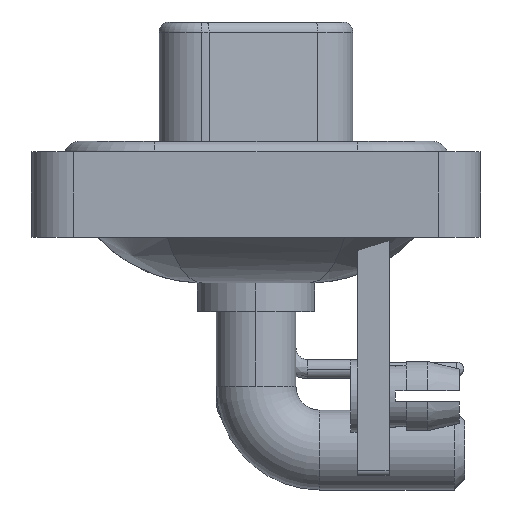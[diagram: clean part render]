
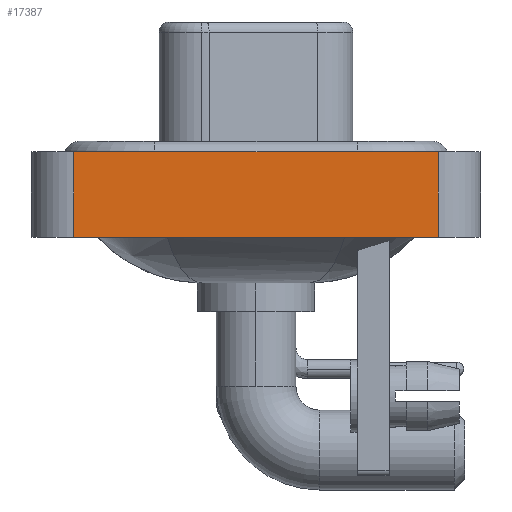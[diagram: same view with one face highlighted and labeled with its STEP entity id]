
A CAD part, left-side view. The second image highlights one B-rep face of the part: STEP entity #17387.
In plain terms, the highlighted planar face has unit normal (-1, 0, 0).
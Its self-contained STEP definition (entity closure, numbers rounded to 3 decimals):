
#965 = LINE ( 'NONE', #7387, #12526 ) ;
#1519 = CARTESIAN_POINT ( 'NONE',  ( -7.3, -8.55, -3.6 ) ) ;
#1933 = DIRECTION ( 'NONE',  ( 0., 0., 1. ) ) ;
#2014 = CARTESIAN_POINT ( 'NONE',  ( -7.3, -8.55, -3.6 ) ) ;
#3002 = CARTESIAN_POINT ( 'NONE',  ( -7.3, 8.55, 0.4 ) ) ;
#3385 = DIRECTION ( 'NONE',  ( 0., 0., 1. ) ) ;
#3701 = LINE ( 'NONE', #9992, #4151 ) ;
#4151 = VECTOR ( 'NONE', #1933, 1000. ) ;
#4696 = CARTESIAN_POINT ( 'NONE',  ( -7.3, 8.55, -3.6 ) ) ;
#4946 = DIRECTION ( 'NONE',  ( 0., -1., 0. ) ) ;
#5593 = AXIS2_PLACEMENT_3D ( 'NONE', #2014, #26640, #16463 ) ;
#7010 = CARTESIAN_POINT ( 'NONE',  ( -7.3, -8.55, 0.4 ) ) ;
#7387 = CARTESIAN_POINT ( 'NONE',  ( -7.3, -8.55, -3.6 ) ) ;
#8001 = VERTEX_POINT ( 'NONE', #3002 ) ;
#8092 = EDGE_CURVE ( 'NONE', #21689, #23166, #24343, .T. ) ;
#9421 = VECTOR ( 'NONE', #3385, 1000. ) ;
#9806 = ORIENTED_EDGE ( 'NONE', *, *, #24217, .F. ) ;
#9937 = PLANE ( 'NONE',  #5593 ) ;
#9992 = CARTESIAN_POINT ( 'NONE',  ( -7.3, 8.55, -3.6 ) ) ;
#12526 = VECTOR ( 'NONE', #21785, 1000. ) ;
#14278 = EDGE_LOOP ( 'NONE', ( #15751, #9806, #25833, #15987 ) ) ;
#15751 = ORIENTED_EDGE ( 'NONE', *, *, #8092, .T. ) ;
#15987 = ORIENTED_EDGE ( 'NONE', *, *, #22024, .T. ) ;
#16463 = DIRECTION ( 'NONE',  ( 0., 0., 1. ) ) ;
#16738 = CARTESIAN_POINT ( 'NONE',  ( -7.3, -8.55, 0.4 ) ) ;
#17387 = ADVANCED_FACE ( 'NONE', ( #18343 ), #9937, .T. ) ;
#18343 = FACE_OUTER_BOUND ( 'NONE', #14278, .T. ) ;
#18893 = VERTEX_POINT ( 'NONE', #4696 ) ;
#21234 = VECTOR ( 'NONE', #4946, 1000. ) ;
#21631 = EDGE_CURVE ( 'NONE', #18893, #8001, #3701, .T. ) ;
#21689 = VERTEX_POINT ( 'NONE', #1519 ) ;
#21785 = DIRECTION ( 'NONE',  ( 0., -1., 0. ) ) ;
#22024 = EDGE_CURVE ( 'NONE', #18893, #21689, #965, .T. ) ;
#23166 = VERTEX_POINT ( 'NONE', #16738 ) ;
#24211 = CARTESIAN_POINT ( 'NONE',  ( -7.3, -8.55, -3.6 ) ) ;
#24217 = EDGE_CURVE ( 'NONE', #8001, #23166, #25637, .T. ) ;
#24343 = LINE ( 'NONE', #24211, #9421 ) ;
#25637 = LINE ( 'NONE', #7010, #21234 ) ;
#25833 = ORIENTED_EDGE ( 'NONE', *, *, #21631, .F. ) ;
#26640 = DIRECTION ( 'NONE',  ( -1., 0., 0. ) ) ;
